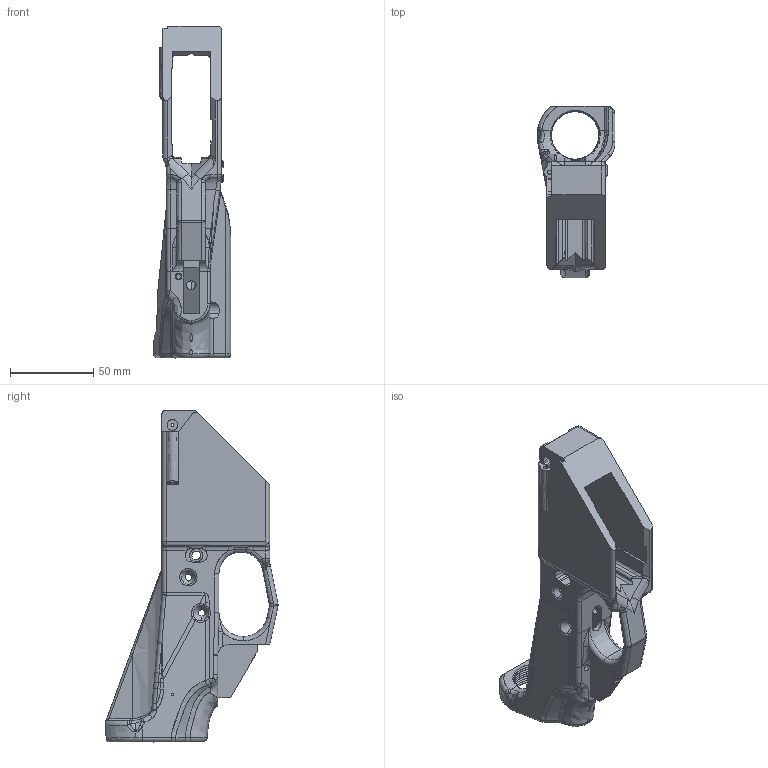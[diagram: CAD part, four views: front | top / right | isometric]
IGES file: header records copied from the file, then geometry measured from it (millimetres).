
Start section: SolidWorks IGES file using analytic representation for surfaces
Global section: file name: AR Lower V3.0.IGS; native system: SolidWorks 2011; preprocessor: SolidWorks 2011; author: Frank; date: 201001.200430; units: inch
Bounding box: 46.72 x 103.45 x 199.48 mm (x, y, z)
Surface area: 60677.9 mm2 (no closed solid volume)
Topology: 0 solids, 0 shells, 753 faces, 9803 edges, 9790 vertices
Faces by surface type: bspline 495, revolution 258
